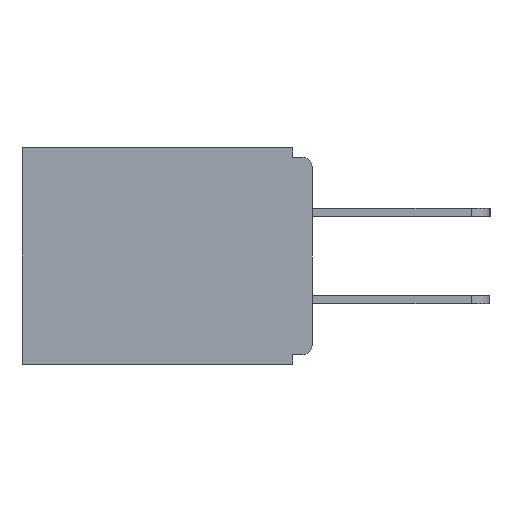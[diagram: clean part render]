
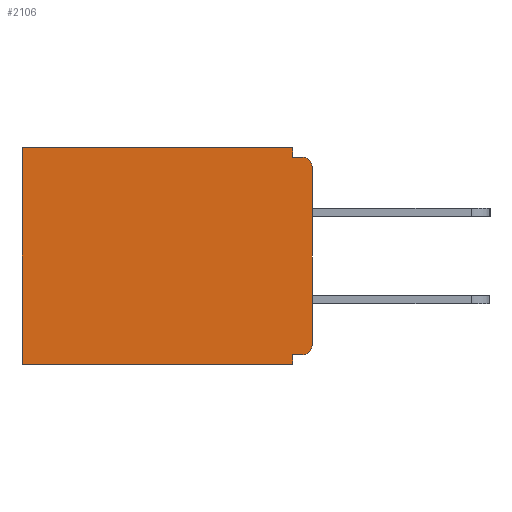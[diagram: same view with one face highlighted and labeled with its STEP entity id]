
A CAD part, left-side view. The second image highlights one B-rep face of the part: STEP entity #2106.
In plain terms, the highlighted planar face has unit normal (-1, 0, 0).
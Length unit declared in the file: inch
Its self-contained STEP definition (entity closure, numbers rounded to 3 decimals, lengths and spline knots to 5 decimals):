
#185 = AXIS2_PLACEMENT_3D ( 'NONE', #17193, #24779, #19297 ) ;
#1202 = EDGE_CURVE ( 'NONE', #20330, #16967, #24700, .T. ) ;
#1559 = DIRECTION ( 'NONE',  ( 0., 0., -1. ) ) ;
#1602 = EDGE_CURVE ( 'NONE', #12011, #5357, #19034, .T. ) ;
#1685 = EDGE_CURVE ( 'NONE', #3441, #23544, #11198, .T. ) ;
#2027 = CARTESIAN_POINT ( 'NONE',  ( 0.298, 0.031, 0. ) ) ;
#2106 = ADVANCED_FACE ( 'NONE', ( #19008 ), #19385, .F. ) ;
#2182 = CARTESIAN_POINT ( 'NONE',  ( 0.298, 0., 0. ) ) ;
#2541 = VERTEX_POINT ( 'NONE', #6791 ) ;
#2695 = VERTEX_POINT ( 'NONE', #6025 ) ;
#3041 = LINE ( 'NONE', #2182, #12421 ) ;
#3320 = ORIENTED_EDGE ( 'NONE', *, *, #1602, .F. ) ;
#3441 = VERTEX_POINT ( 'NONE', #2027 ) ;
#3811 = CARTESIAN_POINT ( 'NONE',  ( 0.298, 0.015, -0.03 ) ) ;
#4387 = VECTOR ( 'NONE', #21203, 39.37008 ) ;
#4400 = EDGE_CURVE ( 'NONE', #23544, #2695, #23027, .T. ) ;
#4513 = AXIS2_PLACEMENT_3D ( 'NONE', #16253, #22604, #18269 ) ;
#5070 = CARTESIAN_POINT ( 'NONE',  ( 0.298, 0.031, -0.343 ) ) ;
#5151 = CARTESIAN_POINT ( 'NONE',  ( 0.298, 0.015, -0.328 ) ) ;
#5357 = VERTEX_POINT ( 'NONE', #17284 ) ;
#5435 = CARTESIAN_POINT ( 'NONE',  ( 0.298, 0., -0.03 ) ) ;
#6025 = CARTESIAN_POINT ( 'NONE',  ( 0.298, 0.015, -0.015 ) ) ;
#6791 = CARTESIAN_POINT ( 'NONE',  ( 0.298, 0.46, 0. ) ) ;
#6976 = DIRECTION ( 'NONE',  ( 0., 0., -1. ) ) ;
#7537 = ORIENTED_EDGE ( 'NONE', *, *, #18268, .T. ) ;
#8074 = DIRECTION ( 'NONE',  ( -1., 0., 0. ) ) ;
#8398 = EDGE_CURVE ( 'NONE', #16967, #12011, #22219, .T. ) ;
#8520 = EDGE_CURVE ( 'NONE', #2541, #5357, #19037, .T. ) ;
#9133 = CARTESIAN_POINT ( 'NONE',  ( 0.298, 0.031, -0.015 ) ) ;
#9365 = CIRCLE ( 'NONE', #4513, 0.015 ) ;
#9747 = CARTESIAN_POINT ( 'NONE',  ( 0.298, 0.031, -0.343 ) ) ;
#11198 = LINE ( 'NONE', #9747, #18392 ) ;
#11637 = DIRECTION ( 'NONE',  ( 0., 0., -1. ) ) ;
#12011 = VERTEX_POINT ( 'NONE', #15513 ) ;
#12252 = AXIS2_PLACEMENT_3D ( 'NONE', #3811, #8074, #22144 ) ;
#12332 = VECTOR ( 'NONE', #24513, 39.37008 ) ;
#12421 = VECTOR ( 'NONE', #13998, 39.37008 ) ;
#13172 = CARTESIAN_POINT ( 'NONE',  ( 0.298, 0.031, -0.328 ) ) ;
#13316 = CARTESIAN_POINT ( 'NONE',  ( 0.298, 0., -0.328 ) ) ;
#13723 = VECTOR ( 'NONE', #23313, 39.37008 ) ;
#13748 = VECTOR ( 'NONE', #19526, 39.37008 ) ;
#13998 = DIRECTION ( 'NONE',  ( 0., 1., 0. ) ) ;
#14283 = ORIENTED_EDGE ( 'NONE', *, *, #1685, .F. ) ;
#14520 = VERTEX_POINT ( 'NONE', #25273 ) ;
#15513 = CARTESIAN_POINT ( 'NONE',  ( 0.298, 0.031, -0.343 ) ) ;
#15700 = LINE ( 'NONE', #17231, #4387 ) ;
#16063 = ORIENTED_EDGE ( 'NONE', *, *, #4400, .F. ) ;
#16241 = EDGE_CURVE ( 'NONE', #17971, #14520, #15700, .T. ) ;
#16253 = CARTESIAN_POINT ( 'NONE',  ( 0.298, 0.015, -0.313 ) ) ;
#16566 = CIRCLE ( 'NONE', #12252, 0.015 ) ;
#16962 = CARTESIAN_POINT ( 'NONE',  ( 0.298, 0., -0.343 ) ) ;
#16967 = VERTEX_POINT ( 'NONE', #13172 ) ;
#17083 = ORIENTED_EDGE ( 'NONE', *, *, #8520, .T. ) ;
#17193 = CARTESIAN_POINT ( 'NONE',  ( 0.298, 0., 0. ) ) ;
#17231 = CARTESIAN_POINT ( 'NONE',  ( 0.298, 0., 0. ) ) ;
#17242 = EDGE_CURVE ( 'NONE', #17971, #2695, #16566, .T. ) ;
#17284 = CARTESIAN_POINT ( 'NONE',  ( 0.298, 0.46, -0.343 ) ) ;
#17971 = VERTEX_POINT ( 'NONE', #5435 ) ;
#18093 = ORIENTED_EDGE ( 'NONE', *, *, #8398, .F. ) ;
#18159 = EDGE_CURVE ( 'NONE', #3441, #2541, #3041, .T. ) ;
#18268 = EDGE_CURVE ( 'NONE', #20330, #14520, #9365, .T. ) ;
#18269 = DIRECTION ( 'NONE',  ( 0., 0., -1. ) ) ;
#18392 = VECTOR ( 'NONE', #1559, 39.37008 ) ;
#18406 = CARTESIAN_POINT ( 'NONE',  ( 0.298, 0., -0.015 ) ) ;
#19008 = FACE_OUTER_BOUND ( 'NONE', #19174, .T. ) ;
#19034 = LINE ( 'NONE', #16962, #13723 ) ;
#19037 = LINE ( 'NONE', #21915, #19685 ) ;
#19174 = EDGE_LOOP ( 'NONE', ( #25977, #16063, #14283, #20692, #17083, #3320, #18093, #21166, #7537, #22234 ) ) ;
#19297 = DIRECTION ( 'NONE',  ( 0., 0., -1. ) ) ;
#19385 = PLANE ( 'NONE',  #185 ) ;
#19526 = DIRECTION ( 'NONE',  ( 0., 1., 0. ) ) ;
#19685 = VECTOR ( 'NONE', #11637, 39.37008 ) ;
#20312 = VECTOR ( 'NONE', #6976, 39.37008 ) ;
#20330 = VERTEX_POINT ( 'NONE', #5151 ) ;
#20692 = ORIENTED_EDGE ( 'NONE', *, *, #18159, .T. ) ;
#21166 = ORIENTED_EDGE ( 'NONE', *, *, #1202, .F. ) ;
#21203 = DIRECTION ( 'NONE',  ( 0., 0., -1. ) ) ;
#21915 = CARTESIAN_POINT ( 'NONE',  ( 0.298, 0.46, 0. ) ) ;
#22144 = DIRECTION ( 'NONE',  ( 0., 0., -1. ) ) ;
#22219 = LINE ( 'NONE', #5070, #20312 ) ;
#22234 = ORIENTED_EDGE ( 'NONE', *, *, #16241, .F. ) ;
#22604 = DIRECTION ( 'NONE',  ( -1., 0., 0. ) ) ;
#23027 = LINE ( 'NONE', #18406, #12332 ) ;
#23313 = DIRECTION ( 'NONE',  ( 0., 1., 0. ) ) ;
#23544 = VERTEX_POINT ( 'NONE', #9133 ) ;
#24513 = DIRECTION ( 'NONE',  ( 0., -1., 0. ) ) ;
#24700 = LINE ( 'NONE', #13316, #13748 ) ;
#24779 = DIRECTION ( 'NONE',  ( 1., 0., 0. ) ) ;
#25273 = CARTESIAN_POINT ( 'NONE',  ( 0.298, 0., -0.313 ) ) ;
#25977 = ORIENTED_EDGE ( 'NONE', *, *, #17242, .T. ) ;
